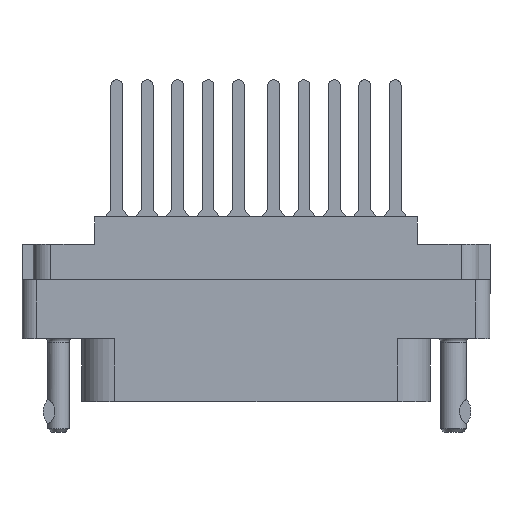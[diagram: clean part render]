
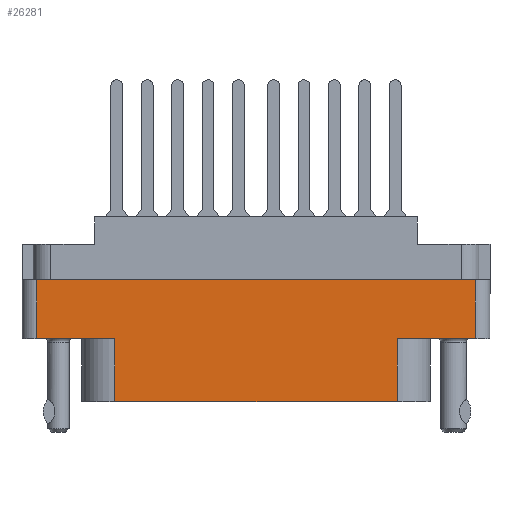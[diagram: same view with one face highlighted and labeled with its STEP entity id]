
A CAD part, front view. The second image highlights one B-rep face of the part: STEP entity #26281.
In plain terms, the highlighted planar face has unit normal (0, -1, 0).
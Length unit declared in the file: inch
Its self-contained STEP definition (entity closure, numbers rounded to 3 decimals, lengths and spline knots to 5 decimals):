
#484 = LINE ( 'NONE', #25719, #14629 ) ;
#540 = LINE ( 'NONE', #25566, #27120 ) ;
#2091 = LINE ( 'NONE', #22115, #24140 ) ;
#2716 = CARTESIAN_POINT ( 'NONE',  ( -1., -0.438, -0.789 ) ) ;
#3251 = DIRECTION ( 'NONE',  ( 1., 0., 0. ) ) ;
#3947 = CARTESIAN_POINT ( 'NONE',  ( -0.604, -0.438, -0.789 ) ) ;
#4128 = CARTESIAN_POINT ( 'NONE',  ( 0.604, -0.438, -0.789 ) ) ;
#4963 = VERTEX_POINT ( 'NONE', #8019 ) ;
#5365 = EDGE_CURVE ( 'NONE', #21750, #25393, #540, .T. ) ;
#5404 = EDGE_CURVE ( 'NONE', #17166, #4963, #6706, .T. ) ;
#5662 = CARTESIAN_POINT ( 'NONE',  ( 0.604, -0.438, -0.52 ) ) ;
#6413 = CARTESIAN_POINT ( 'NONE',  ( 0., -0.438, -0.268 ) ) ;
#6497 = LINE ( 'NONE', #25394, #35321 ) ;
#6706 = LINE ( 'NONE', #22561, #15230 ) ;
#7185 = EDGE_CURVE ( 'NONE', #25393, #43092, #2091, .T. ) ;
#7602 = EDGE_CURVE ( 'NONE', #17166, #43092, #32572, .T. ) ;
#8019 = CARTESIAN_POINT ( 'NONE',  ( 0.938, -0.438, -0.268 ) ) ;
#10818 = DIRECTION ( 'NONE',  ( -1., 0., 0. ) ) ;
#11165 = DIRECTION ( 'NONE',  ( 1., 0., 0. ) ) ;
#11905 = FACE_OUTER_BOUND ( 'NONE', #36932, .T. ) ;
#14527 = DIRECTION ( 'NONE',  ( 0., 0., 1. ) ) ;
#14629 = VECTOR ( 'NONE', #19084, 39.37008 ) ;
#15230 = VECTOR ( 'NONE', #22726, 39.37008 ) ;
#17015 = ORIENTED_EDGE ( 'NONE', *, *, #46120, .T. ) ;
#17166 = VERTEX_POINT ( 'NONE', #28848 ) ;
#17812 = ORIENTED_EDGE ( 'NONE', *, *, #21029, .T. ) ;
#17889 = VERTEX_POINT ( 'NONE', #43461 ) ;
#19084 = DIRECTION ( 'NONE',  ( 1., 0., 0. ) ) ;
#19215 = CARTESIAN_POINT ( 'NONE',  ( -0.938, -0.438, -0.52 ) ) ;
#19449 = LINE ( 'NONE', #6413, #34712 ) ;
#19694 = ORIENTED_EDGE ( 'NONE', *, *, #27168, .T. ) ;
#19695 = ORIENTED_EDGE ( 'NONE', *, *, #7185, .T. ) ;
#21014 = ORIENTED_EDGE ( 'NONE', *, *, #7602, .F. ) ;
#21029 = EDGE_CURVE ( 'NONE', #17889, #21750, #24750, .T. ) ;
#21750 = VERTEX_POINT ( 'NONE', #22669 ) ;
#21902 = DIRECTION ( 'NONE',  ( 0., 0., -1. ) ) ;
#22115 = CARTESIAN_POINT ( 'NONE',  ( 0.604, -0.438, -0.52 ) ) ;
#22561 = CARTESIAN_POINT ( 'NONE',  ( 0.938, -0.438, -0.789 ) ) ;
#22669 = CARTESIAN_POINT ( 'NONE',  ( -0.604, -0.438, -0.789 ) ) ;
#22726 = DIRECTION ( 'NONE',  ( 0., 0., 1. ) ) ;
#24140 = VECTOR ( 'NONE', #14527, 39.37008 ) ;
#24567 = EDGE_CURVE ( 'NONE', #45220, #4963, #19449, .T. ) ;
#24750 = LINE ( 'NONE', #3947, #28687 ) ;
#25223 = ORIENTED_EDGE ( 'NONE', *, *, #5365, .T. ) ;
#25393 = VERTEX_POINT ( 'NONE', #4128 ) ;
#25394 = CARTESIAN_POINT ( 'NONE',  ( -0.938, -0.438, -0.789 ) ) ;
#25566 = CARTESIAN_POINT ( 'NONE',  ( -1., -0.438, -0.789 ) ) ;
#25719 = CARTESIAN_POINT ( 'NONE',  ( 0., -0.438, -0.52 ) ) ;
#26281 = ADVANCED_FACE ( 'NONE', ( #11905 ), #31945, .T. ) ;
#26482 = ORIENTED_EDGE ( 'NONE', *, *, #5404, .T. ) ;
#27120 = VECTOR ( 'NONE', #11165, 39.37008 ) ;
#27168 = EDGE_CURVE ( 'NONE', #45220, #30410, #6497, .T. ) ;
#28687 = VECTOR ( 'NONE', #36080, 39.37008 ) ;
#28692 = CARTESIAN_POINT ( 'NONE',  ( 0., -0.438, -0.52 ) ) ;
#28848 = CARTESIAN_POINT ( 'NONE',  ( 0.938, -0.438, -0.52 ) ) ;
#28932 = DIRECTION ( 'NONE',  ( 0., 0., -1. ) ) ;
#29535 = CARTESIAN_POINT ( 'NONE',  ( -0.938, -0.438, -0.268 ) ) ;
#30083 = AXIS2_PLACEMENT_3D ( 'NONE', #2716, #39730, #28932 ) ;
#30309 = VECTOR ( 'NONE', #10818, 39.37008 ) ;
#30410 = VERTEX_POINT ( 'NONE', #19215 ) ;
#31945 = PLANE ( 'NONE',  #30083 ) ;
#32572 = LINE ( 'NONE', #28692, #30309 ) ;
#33946 = ORIENTED_EDGE ( 'NONE', *, *, #24567, .F. ) ;
#34712 = VECTOR ( 'NONE', #3251, 39.37008 ) ;
#35321 = VECTOR ( 'NONE', #21902, 39.37008 ) ;
#36080 = DIRECTION ( 'NONE',  ( 0., 0., -1. ) ) ;
#36932 = EDGE_LOOP ( 'NONE', ( #33946, #19694, #17015, #17812, #25223, #19695, #21014, #26482 ) ) ;
#39730 = DIRECTION ( 'NONE',  ( 0., -1., 0. ) ) ;
#43092 = VERTEX_POINT ( 'NONE', #5662 ) ;
#43461 = CARTESIAN_POINT ( 'NONE',  ( -0.604, -0.438, -0.52 ) ) ;
#45220 = VERTEX_POINT ( 'NONE', #29535 ) ;
#46120 = EDGE_CURVE ( 'NONE', #30410, #17889, #484, .T. ) ;
